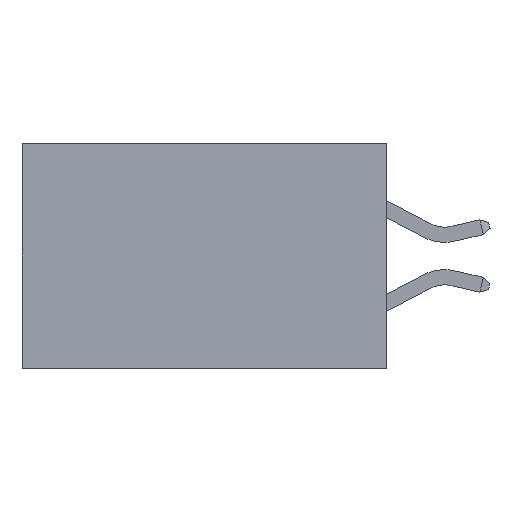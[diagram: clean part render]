
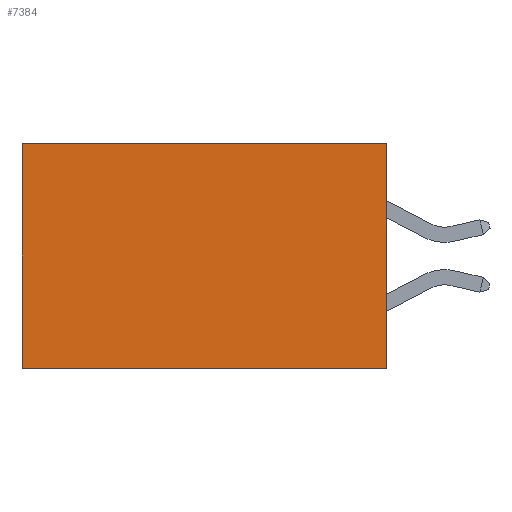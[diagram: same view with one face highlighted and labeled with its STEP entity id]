
A CAD part, left-side view. The second image highlights one B-rep face of the part: STEP entity #7384.
In plain terms, the highlighted planar face has unit normal (-1, 0, 0).
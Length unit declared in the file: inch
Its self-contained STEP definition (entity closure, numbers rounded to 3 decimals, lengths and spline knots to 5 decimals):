
#361 = VERTEX_POINT ( 'NONE', #5868 ) ;
#472 = VERTEX_POINT ( 'NONE', #25201 ) ;
#772 = EDGE_CURVE ( 'NONE', #22728, #472, #5926, .T. ) ;
#2476 = VECTOR ( 'NONE', #22510, 39.37008 ) ;
#3215 = PLANE ( 'NONE',  #22399 ) ;
#3475 = VECTOR ( 'NONE', #24991, 39.37008 ) ;
#4310 = DIRECTION ( 'NONE',  ( 0., 0., -1. ) ) ;
#4481 = VERTEX_POINT ( 'NONE', #21485 ) ;
#5868 = CARTESIAN_POINT ( 'NONE',  ( 0.298, 0.6, 0. ) ) ;
#5926 = LINE ( 'NONE', #18041, #11667 ) ;
#7384 = ADVANCED_FACE ( 'NONE', ( #9630 ), #3215, .F. ) ;
#7714 = CARTESIAN_POINT ( 'NONE',  ( 0.298, 0., -0.37 ) ) ;
#8394 = EDGE_CURVE ( 'NONE', #361, #4481, #20776, .T. ) ;
#8447 = CARTESIAN_POINT ( 'NONE',  ( 0.298, 0., 0. ) ) ;
#9511 = ORIENTED_EDGE ( 'NONE', *, *, #8394, .T. ) ;
#9630 = FACE_OUTER_BOUND ( 'NONE', #10874, .T. ) ;
#10874 = EDGE_LOOP ( 'NONE', ( #9511, #27305, #27492, #26148 ) ) ;
#11667 = VECTOR ( 'NONE', #21379, 39.37008 ) ;
#11925 = DIRECTION ( 'NONE',  ( 1., 0., 0. ) ) ;
#13923 = EDGE_CURVE ( 'NONE', #22728, #361, #13987, .T. ) ;
#13987 = LINE ( 'NONE', #24656, #2476 ) ;
#17307 = CARTESIAN_POINT ( 'NONE',  ( 0.298, 0.6, 0. ) ) ;
#18041 = CARTESIAN_POINT ( 'NONE',  ( 0.298, 0., 0. ) ) ;
#20776 = LINE ( 'NONE', #17307, #27052 ) ;
#21379 = DIRECTION ( 'NONE',  ( 0., 0., -1. ) ) ;
#21485 = CARTESIAN_POINT ( 'NONE',  ( 0.298, 0.6, -0.37 ) ) ;
#22399 = AXIS2_PLACEMENT_3D ( 'NONE', #26874, #11925, #26968 ) ;
#22510 = DIRECTION ( 'NONE',  ( 0., 1., 0. ) ) ;
#22728 = VERTEX_POINT ( 'NONE', #8447 ) ;
#24476 = EDGE_CURVE ( 'NONE', #472, #4481, #27080, .T. ) ;
#24656 = CARTESIAN_POINT ( 'NONE',  ( 0.298, 0., 0. ) ) ;
#24991 = DIRECTION ( 'NONE',  ( 0., 1., 0. ) ) ;
#25201 = CARTESIAN_POINT ( 'NONE',  ( 0.298, 0., -0.37 ) ) ;
#26148 = ORIENTED_EDGE ( 'NONE', *, *, #13923, .T. ) ;
#26874 = CARTESIAN_POINT ( 'NONE',  ( 0.298, 0., 0. ) ) ;
#26968 = DIRECTION ( 'NONE',  ( 0., 0., -1. ) ) ;
#27052 = VECTOR ( 'NONE', #4310, 39.37008 ) ;
#27080 = LINE ( 'NONE', #7714, #3475 ) ;
#27305 = ORIENTED_EDGE ( 'NONE', *, *, #24476, .F. ) ;
#27492 = ORIENTED_EDGE ( 'NONE', *, *, #772, .F. ) ;
